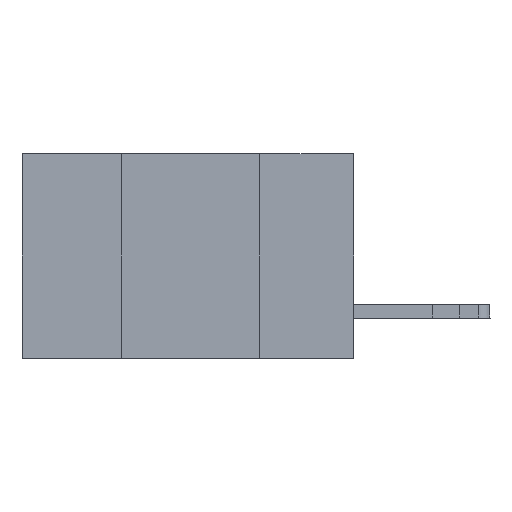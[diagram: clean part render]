
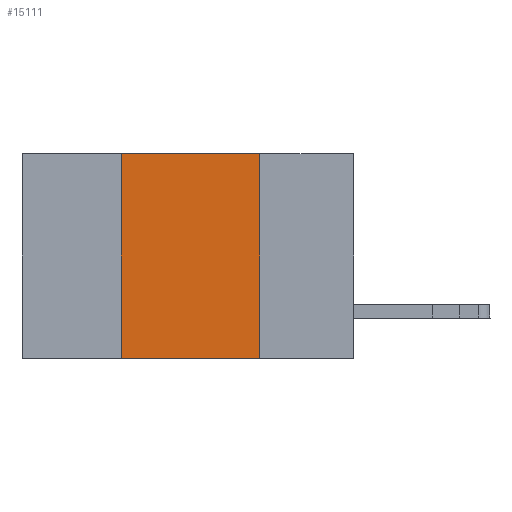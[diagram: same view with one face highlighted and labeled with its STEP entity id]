
A CAD part, left-side view. The second image highlights one B-rep face of the part: STEP entity #15111.
In plain terms, the highlighted planar face has unit normal (-1, 0, 0).
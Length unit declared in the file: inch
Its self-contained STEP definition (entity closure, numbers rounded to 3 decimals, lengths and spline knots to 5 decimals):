
#312 = CARTESIAN_POINT ( 'NONE',  ( 0., 0.6, 0. ) ) ;
#1128 = EDGE_LOOP ( 'NONE', ( #8842, #19878, #29294, #11066 ) ) ;
#1232 = VERTEX_POINT ( 'NONE', #22215 ) ;
#1373 = CARTESIAN_POINT ( 'NONE',  ( 0., 0.17, 0. ) ) ;
#1889 = EDGE_CURVE ( 'NONE', #1232, #18641, #35999, .T. ) ;
#3206 = CARTESIAN_POINT ( 'NONE',  ( 0., 0.42, 0. ) ) ;
#3346 = DIRECTION ( 'NONE',  ( 1., 0., 0. ) ) ;
#3971 = CARTESIAN_POINT ( 'NONE',  ( 0., 0.6, -0.37 ) ) ;
#5885 = EDGE_CURVE ( 'NONE', #16829, #18641, #36607, .T. ) ;
#8842 = ORIENTED_EDGE ( 'NONE', *, *, #5885, .F. ) ;
#9995 = DIRECTION ( 'NONE',  ( 0., -1., 0. ) ) ;
#11066 = ORIENTED_EDGE ( 'NONE', *, *, #1889, .T. ) ;
#11976 = CARTESIAN_POINT ( 'NONE',  ( 0., 0.17, 0. ) ) ;
#12433 = FACE_OUTER_BOUND ( 'NONE', #1128, .T. ) ;
#12845 = DIRECTION ( 'NONE',  ( 0., -1., 0. ) ) ;
#13833 = LINE ( 'NONE', #36155, #15676 ) ;
#15111 = ADVANCED_FACE ( 'NONE', ( #12433 ), #35426, .F. ) ;
#15282 = EDGE_CURVE ( 'NONE', #25951, #16829, #13833, .T. ) ;
#15676 = VECTOR ( 'NONE', #9995, 39.37008 ) ;
#16829 = VERTEX_POINT ( 'NONE', #1373 ) ;
#18641 = VERTEX_POINT ( 'NONE', #36262 ) ;
#19878 = ORIENTED_EDGE ( 'NONE', *, *, #15282, .F. ) ;
#20251 = AXIS2_PLACEMENT_3D ( 'NONE', #312, #3346, #23864 ) ;
#20373 = VECTOR ( 'NONE', #20803, 39.37008 ) ;
#20640 = VECTOR ( 'NONE', #12845, 39.37008 ) ;
#20803 = DIRECTION ( 'NONE',  ( 0., 0., -1. ) ) ;
#22215 = CARTESIAN_POINT ( 'NONE',  ( 0., 0.42, -0.37 ) ) ;
#23122 = VECTOR ( 'NONE', #26218, 39.37008 ) ;
#23864 = DIRECTION ( 'NONE',  ( 0., 0., -1. ) ) ;
#25951 = VERTEX_POINT ( 'NONE', #3206 ) ;
#26218 = DIRECTION ( 'NONE',  ( 0., 0., 1. ) ) ;
#29294 = ORIENTED_EDGE ( 'NONE', *, *, #30104, .F. ) ;
#30104 = EDGE_CURVE ( 'NONE', #1232, #25951, #30850, .T. ) ;
#30850 = LINE ( 'NONE', #34839, #23122 ) ;
#34839 = CARTESIAN_POINT ( 'NONE',  ( 0., 0.42, 0. ) ) ;
#35426 = PLANE ( 'NONE',  #20251 ) ;
#35999 = LINE ( 'NONE', #3971, #20640 ) ;
#36155 = CARTESIAN_POINT ( 'NONE',  ( 0., 0.6, 0. ) ) ;
#36262 = CARTESIAN_POINT ( 'NONE',  ( 0., 0.17, -0.37 ) ) ;
#36607 = LINE ( 'NONE', #11976, #20373 ) ;
